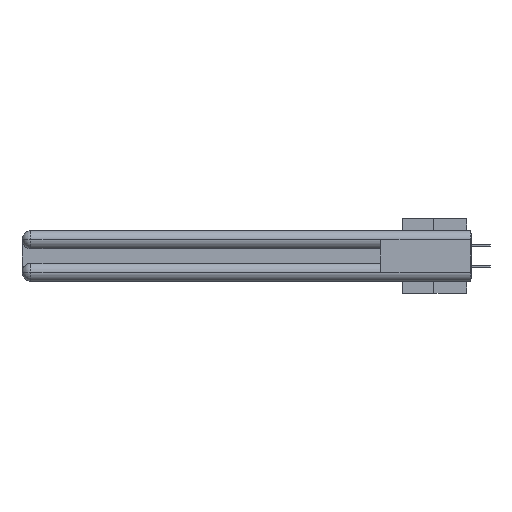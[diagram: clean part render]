
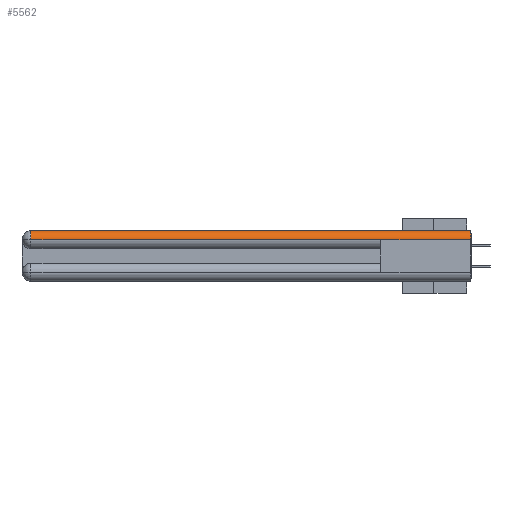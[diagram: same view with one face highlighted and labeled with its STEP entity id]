
A CAD part, left-side view. The second image highlights one B-rep face of the part: STEP entity #5562.
In plain terms, the highlighted cylindrical face has radius 1.562 mm (diameter 3.124 mm), a partial arc.
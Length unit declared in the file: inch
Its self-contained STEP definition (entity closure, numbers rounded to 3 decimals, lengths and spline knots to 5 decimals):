
#1314 = ORIENTED_EDGE ( 'NONE', *, *, #8926, .F. ) ;
#2179 = CARTESIAN_POINT ( 'NONE',  ( 0.0615, 0., 0. ) ) ;
#2279 = EDGE_LOOP ( 'NONE', ( #1314, #10806, #34758, #10003, #33607 ) ) ;
#2756 = AXIS2_PLACEMENT_3D ( 'NONE', #22859, #22728, #22991 ) ;
#3115 = DIRECTION ( 'NONE',  ( 0., -1., 0. ) ) ;
#4392 = LINE ( 'NONE', #17317, #32433 ) ;
#5489 = CIRCLE ( 'NONE', #23721, 0.0615 ) ;
#5562 = ADVANCED_FACE ( 'NONE', ( #9855 ), #16564, .T. ) ;
#6288 = VERTEX_POINT ( 'NONE', #8209 ) ;
#8209 = CARTESIAN_POINT ( 'NONE',  ( 0., 0.6, -0.0615 ) ) ;
#8547 = LINE ( 'NONE', #2179, #13319 ) ;
#8926 = EDGE_CURVE ( 'NONE', #17212, #37418, #8547, .T. ) ;
#9855 = FACE_OUTER_BOUND ( 'NONE', #2279, .T. ) ;
#10003 = ORIENTED_EDGE ( 'NONE', *, *, #25718, .F. ) ;
#10806 = ORIENTED_EDGE ( 'NONE', *, *, #30685, .T. ) ;
#12930 = CARTESIAN_POINT ( 'NONE',  ( 0., 3., -0.0615 ) ) ;
#12962 = CARTESIAN_POINT ( 'NONE',  ( 0.0615, 0., -0.0615 ) ) ;
#13319 = VECTOR ( 'NONE', #18045, 39.37008 ) ;
#14939 = DIRECTION ( 'NONE',  ( 0., 0., 1. ) ) ;
#16365 = EDGE_CURVE ( 'NONE', #19808, #6288, #33649, .T. ) ;
#16564 = CYLINDRICAL_SURFACE ( 'NONE', #2756, 0.0615 ) ;
#17212 = VERTEX_POINT ( 'NONE', #29204 ) ;
#17317 = CARTESIAN_POINT ( 'NONE',  ( 0., 3., -0.0615 ) ) ;
#18045 = DIRECTION ( 'NONE',  ( 0., -1., 0. ) ) ;
#19285 = VERTEX_POINT ( 'NONE', #29389 ) ;
#19393 = DIRECTION ( 'NONE',  ( 1., 0., 0. ) ) ;
#19808 = VERTEX_POINT ( 'NONE', #19932 ) ;
#19850 = CIRCLE ( 'NONE', #23256, 0.0615 ) ;
#19932 = CARTESIAN_POINT ( 'NONE',  ( 0., 2.94, -0.0615 ) ) ;
#22728 = DIRECTION ( 'NONE',  ( 0., 1., 0. ) ) ;
#22859 = CARTESIAN_POINT ( 'NONE',  ( 0.0615, 0., -0.0615 ) ) ;
#22991 = DIRECTION ( 'NONE',  ( 0., 0., 1. ) ) ;
#23256 = AXIS2_PLACEMENT_3D ( 'NONE', #39241, #3115, #14939 ) ;
#23420 = DIRECTION ( 'NONE',  ( 0., 1., 0. ) ) ;
#23721 = AXIS2_PLACEMENT_3D ( 'NONE', #12962, #25117, #19393 ) ;
#25117 = DIRECTION ( 'NONE',  ( 0., -1., 0. ) ) ;
#25592 = VECTOR ( 'NONE', #38029, 39.37008 ) ;
#25718 = EDGE_CURVE ( 'NONE', #19285, #6288, #4392, .T. ) ;
#26494 = CARTESIAN_POINT ( 'NONE',  ( 0.0615, 0., 0. ) ) ;
#29204 = CARTESIAN_POINT ( 'NONE',  ( 0.0615, 2.94, 0. ) ) ;
#29389 = CARTESIAN_POINT ( 'NONE',  ( 0., 0., -0.0615 ) ) ;
#29850 = EDGE_CURVE ( 'NONE', #37418, #19285, #5489, .T. ) ;
#30685 = EDGE_CURVE ( 'NONE', #17212, #19808, #19850, .T. ) ;
#32433 = VECTOR ( 'NONE', #23420, 39.37008 ) ;
#33607 = ORIENTED_EDGE ( 'NONE', *, *, #29850, .F. ) ;
#33649 = LINE ( 'NONE', #12930, #25592 ) ;
#34758 = ORIENTED_EDGE ( 'NONE', *, *, #16365, .T. ) ;
#37418 = VERTEX_POINT ( 'NONE', #26494 ) ;
#38029 = DIRECTION ( 'NONE',  ( 0., -1., 0. ) ) ;
#39241 = CARTESIAN_POINT ( 'NONE',  ( 0.0615, 2.94, -0.0615 ) ) ;
